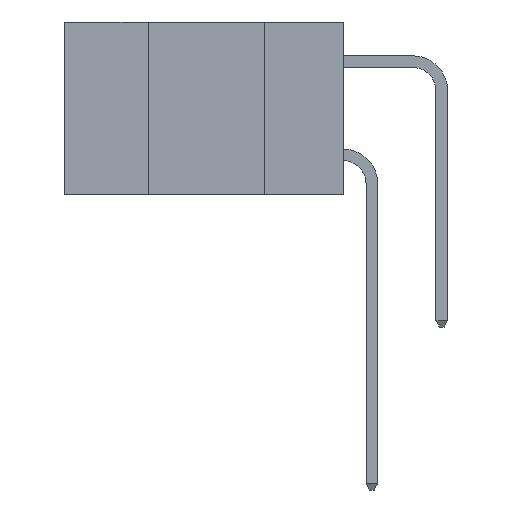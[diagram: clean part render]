
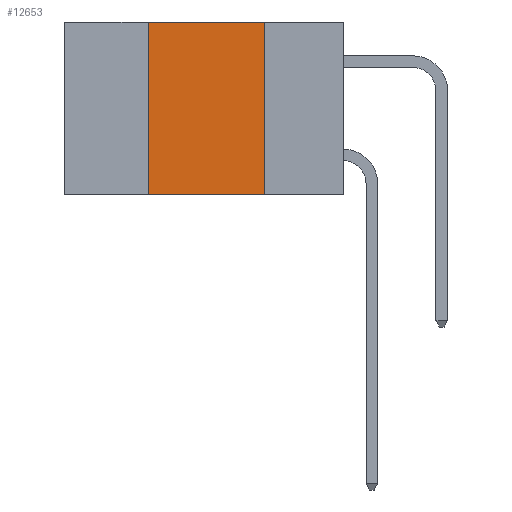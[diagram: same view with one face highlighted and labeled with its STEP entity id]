
A CAD part, left-side view. The second image highlights one B-rep face of the part: STEP entity #12653.
In plain terms, the highlighted planar face has unit normal (-1, 0, 0).
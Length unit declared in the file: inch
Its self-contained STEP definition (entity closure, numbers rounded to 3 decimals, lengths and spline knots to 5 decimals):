
#57 = PLANE ( 'NONE',  #18046 ) ;
#1248 = EDGE_LOOP ( 'NONE', ( #1390, #18774, #12358, #6837 ) ) ;
#1390 = ORIENTED_EDGE ( 'NONE', *, *, #3435, .F. ) ;
#1686 = DIRECTION ( 'NONE',  ( 1., 0., 0. ) ) ;
#1827 = CARTESIAN_POINT ( 'NONE',  ( 0., 0.17, 0. ) ) ;
#2381 = EDGE_CURVE ( 'NONE', #19403, #2574, #18755, .T. ) ;
#2574 = VERTEX_POINT ( 'NONE', #1827 ) ;
#3435 = EDGE_CURVE ( 'NONE', #2574, #16912, #9233, .T. ) ;
#4429 = CARTESIAN_POINT ( 'NONE',  ( 0., 0.42, -0.37 ) ) ;
#5839 = LINE ( 'NONE', #4429, #13609 ) ;
#6614 = EDGE_CURVE ( 'NONE', #19868, #16912, #8623, .T. ) ;
#6837 = ORIENTED_EDGE ( 'NONE', *, *, #6614, .T. ) ;
#7508 = CARTESIAN_POINT ( 'NONE',  ( 0., 0.17, -0.37 ) ) ;
#8623 = LINE ( 'NONE', #11015, #16371 ) ;
#9233 = LINE ( 'NONE', #14697, #16505 ) ;
#9996 = VECTOR ( 'NONE', #14798, 39.37008 ) ;
#10206 = FACE_OUTER_BOUND ( 'NONE', #1248, .T. ) ;
#10926 = DIRECTION ( 'NONE',  ( 0., -1., 0. ) ) ;
#11015 = CARTESIAN_POINT ( 'NONE',  ( 0., 0.6, -0.37 ) ) ;
#11038 = CARTESIAN_POINT ( 'NONE',  ( 0., 0.6, 0. ) ) ;
#12358 = ORIENTED_EDGE ( 'NONE', *, *, #13195, .F. ) ;
#12598 = DIRECTION ( 'NONE',  ( 0., 0., -1. ) ) ;
#12653 = ADVANCED_FACE ( 'NONE', ( #10206 ), #57, .F. ) ;
#12749 = CARTESIAN_POINT ( 'NONE',  ( 0., 0.42, 0. ) ) ;
#13195 = EDGE_CURVE ( 'NONE', #19868, #19403, #5839, .T. ) ;
#13609 = VECTOR ( 'NONE', #18487, 39.37008 ) ;
#14603 = DIRECTION ( 'NONE',  ( 0., 0., -1. ) ) ;
#14697 = CARTESIAN_POINT ( 'NONE',  ( 0., 0.17, -0.37 ) ) ;
#14798 = DIRECTION ( 'NONE',  ( 0., -1., 0. ) ) ;
#16371 = VECTOR ( 'NONE', #10926, 39.37008 ) ;
#16505 = VECTOR ( 'NONE', #14603, 39.37008 ) ;
#16912 = VERTEX_POINT ( 'NONE', #7508 ) ;
#17996 = CARTESIAN_POINT ( 'NONE',  ( 0., 0.6, 0. ) ) ;
#18046 = AXIS2_PLACEMENT_3D ( 'NONE', #11038, #1686, #12598 ) ;
#18487 = DIRECTION ( 'NONE',  ( 0., 0., 1. ) ) ;
#18755 = LINE ( 'NONE', #17996, #9996 ) ;
#18774 = ORIENTED_EDGE ( 'NONE', *, *, #2381, .F. ) ;
#19403 = VERTEX_POINT ( 'NONE', #12749 ) ;
#19868 = VERTEX_POINT ( 'NONE', #19979 ) ;
#19979 = CARTESIAN_POINT ( 'NONE',  ( 0., 0.42, -0.37 ) ) ;
